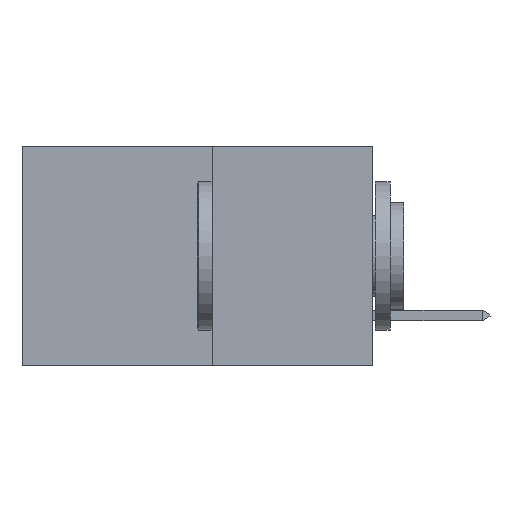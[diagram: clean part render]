
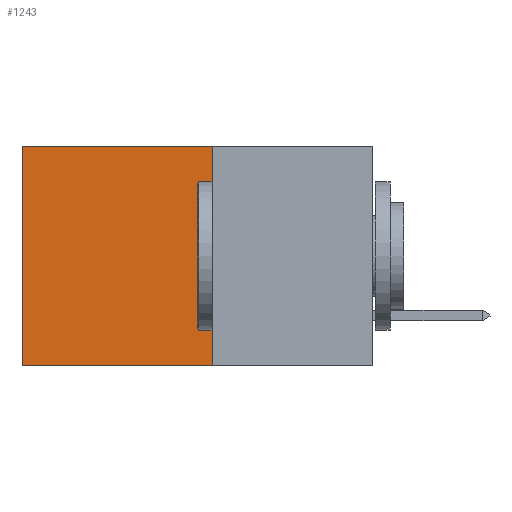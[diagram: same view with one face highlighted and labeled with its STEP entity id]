
A CAD part, left-side view. The second image highlights one B-rep face of the part: STEP entity #1243.
In plain terms, the highlighted planar face has unit normal (-1, 0, 0).
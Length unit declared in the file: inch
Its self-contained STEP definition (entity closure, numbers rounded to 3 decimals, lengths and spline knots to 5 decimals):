
#20 = EDGE_CURVE ( 'NONE', #5978, #9195, #6006, .T. ) ;
#294 = AXIS2_PLACEMENT_3D ( 'NONE', #5240, #9734, #9680 ) ;
#643 = EDGE_CURVE ( 'NONE', #5978, #8685, #1950, .T. ) ;
#699 = ORIENTED_EDGE ( 'NONE', *, *, #5615, .T. ) ;
#1243 = ADVANCED_FACE ( 'NONE', ( #4803 ), #7556, .F. ) ;
#1503 = EDGE_CURVE ( 'NONE', #9195, #9567, #2420, .T. ) ;
#1598 = ORIENTED_EDGE ( 'NONE', *, *, #643, .T. ) ;
#1738 = CARTESIAN_POINT ( 'NONE',  ( 0.277, 0.27, 0. ) ) ;
#1871 = LINE ( 'NONE', #2464, #7875 ) ;
#1873 = CARTESIAN_POINT ( 'NONE',  ( 0.277, 0.27, -0.37 ) ) ;
#1950 = LINE ( 'NONE', #1738, #9678 ) ;
#2203 = VECTOR ( 'NONE', #3345, 39.37008 ) ;
#2420 = LINE ( 'NONE', #6697, #6448 ) ;
#2464 = CARTESIAN_POINT ( 'NONE',  ( 0.277, 0.59, -0.37 ) ) ;
#3165 = ORIENTED_EDGE ( 'NONE', *, *, #1503, .F. ) ;
#3166 = CARTESIAN_POINT ( 'NONE',  ( 0.277, 0.59, -0.37 ) ) ;
#3345 = DIRECTION ( 'NONE',  ( 0., 0., -1. ) ) ;
#3670 = CARTESIAN_POINT ( 'NONE',  ( 0.277, 0.27, 0. ) ) ;
#4638 = ORIENTED_EDGE ( 'NONE', *, *, #20, .F. ) ;
#4803 = FACE_OUTER_BOUND ( 'NONE', #5246, .T. ) ;
#5240 = CARTESIAN_POINT ( 'NONE',  ( 0.277, 0.27, -0.37 ) ) ;
#5246 = EDGE_LOOP ( 'NONE', ( #699, #3165, #4638, #1598 ) ) ;
#5615 = EDGE_CURVE ( 'NONE', #8685, #9567, #1871, .T. ) ;
#5978 = VERTEX_POINT ( 'NONE', #3670 ) ;
#6006 = LINE ( 'NONE', #8846, #2203 ) ;
#6298 = CARTESIAN_POINT ( 'NONE',  ( 0.277, 0.59, 0. ) ) ;
#6448 = VECTOR ( 'NONE', #7930, 39.37008 ) ;
#6697 = CARTESIAN_POINT ( 'NONE',  ( 0.277, 0.27, -0.37 ) ) ;
#6984 = DIRECTION ( 'NONE',  ( 0., 0., -1. ) ) ;
#7217 = DIRECTION ( 'NONE',  ( 0., 1., 0. ) ) ;
#7556 = PLANE ( 'NONE',  #294 ) ;
#7875 = VECTOR ( 'NONE', #6984, 39.37008 ) ;
#7930 = DIRECTION ( 'NONE',  ( 0., 1., 0. ) ) ;
#8685 = VERTEX_POINT ( 'NONE', #6298 ) ;
#8846 = CARTESIAN_POINT ( 'NONE',  ( 0.277, 0.27, -0.37 ) ) ;
#9195 = VERTEX_POINT ( 'NONE', #1873 ) ;
#9567 = VERTEX_POINT ( 'NONE', #3166 ) ;
#9678 = VECTOR ( 'NONE', #7217, 39.37008 ) ;
#9680 = DIRECTION ( 'NONE',  ( 0., 0., -1. ) ) ;
#9734 = DIRECTION ( 'NONE',  ( 1., 0., 0. ) ) ;
